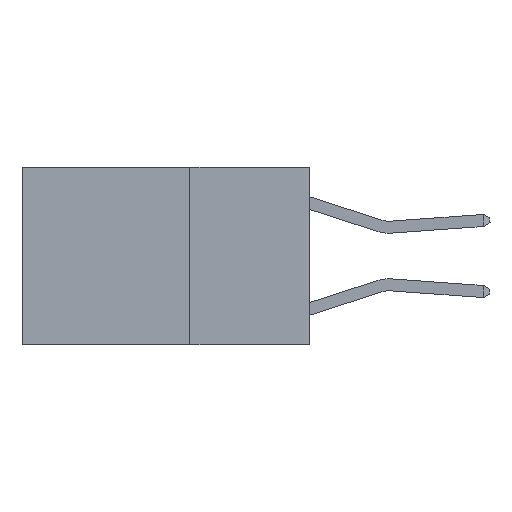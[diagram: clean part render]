
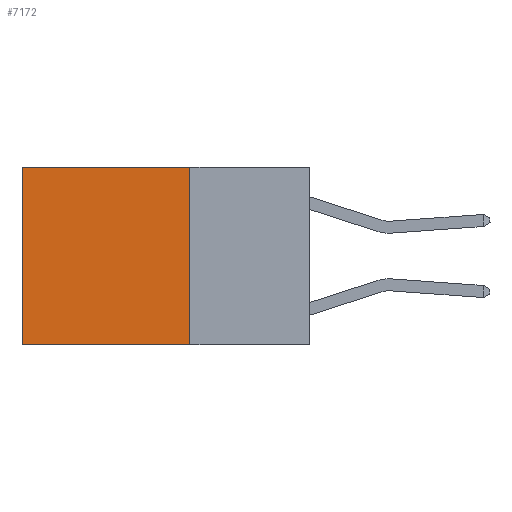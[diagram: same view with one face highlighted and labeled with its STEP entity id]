
A CAD part, left-side view. The second image highlights one B-rep face of the part: STEP entity #7172.
In plain terms, the highlighted planar face has unit normal (-1, 0, 0).
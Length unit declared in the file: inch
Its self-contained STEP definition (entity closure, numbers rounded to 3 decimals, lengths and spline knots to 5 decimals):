
#944 = ORIENTED_EDGE ( 'NONE', *, *, #3419, .T. ) ;
#1296 = LINE ( 'NONE', #1952, #4700 ) ;
#1952 = CARTESIAN_POINT ( 'NONE',  ( 0.2625, 0.25, 0. ) ) ;
#2015 = ORIENTED_EDGE ( 'NONE', *, *, #5008, .F. ) ;
#2053 = EDGE_CURVE ( 'NONE', #6786, #6449, #12035, .T. ) ;
#2470 = DIRECTION ( 'NONE',  ( 1., 0., 0. ) ) ;
#3419 = EDGE_CURVE ( 'NONE', #17197, #6449, #12396, .T. ) ;
#3831 = ORIENTED_EDGE ( 'NONE', *, *, #2053, .F. ) ;
#4368 = VERTEX_POINT ( 'NONE', #16659 ) ;
#4700 = VECTOR ( 'NONE', #11800, 39.37008 ) ;
#4838 = DIRECTION ( 'NONE',  ( 0., 0., -1. ) ) ;
#5008 = EDGE_CURVE ( 'NONE', #4368, #6786, #13356, .T. ) ;
#6449 = VERTEX_POINT ( 'NONE', #8469 ) ;
#6786 = VERTEX_POINT ( 'NONE', #12596 ) ;
#7172 = ADVANCED_FACE ( 'NONE', ( #14935 ), #10986, .F. ) ;
#8469 = CARTESIAN_POINT ( 'NONE',  ( 0.2625, 0.6, -0.37 ) ) ;
#9578 = EDGE_CURVE ( 'NONE', #4368, #17197, #1296, .T. ) ;
#9776 = AXIS2_PLACEMENT_3D ( 'NONE', #14959, #2470, #12339 ) ;
#10275 = ORIENTED_EDGE ( 'NONE', *, *, #9578, .T. ) ;
#10650 = CARTESIAN_POINT ( 'NONE',  ( 0.2625, 0.25, 0. ) ) ;
#10986 = PLANE ( 'NONE',  #9776 ) ;
#11800 = DIRECTION ( 'NONE',  ( 0., 1., 0. ) ) ;
#11935 = CARTESIAN_POINT ( 'NONE',  ( 0.2625, 0.25, -0.37 ) ) ;
#12035 = LINE ( 'NONE', #11935, #15172 ) ;
#12339 = DIRECTION ( 'NONE',  ( 0., 0., -1. ) ) ;
#12396 = LINE ( 'NONE', #14474, #16318 ) ;
#12596 = CARTESIAN_POINT ( 'NONE',  ( 0.2625, 0.25, -0.37 ) ) ;
#13356 = LINE ( 'NONE', #10650, #16847 ) ;
#14474 = CARTESIAN_POINT ( 'NONE',  ( 0.2625, 0.6, 0. ) ) ;
#14495 = EDGE_LOOP ( 'NONE', ( #944, #3831, #2015, #10275 ) ) ;
#14935 = FACE_OUTER_BOUND ( 'NONE', #14495, .T. ) ;
#14959 = CARTESIAN_POINT ( 'NONE',  ( 0.2625, 0.25, 0. ) ) ;
#15172 = VECTOR ( 'NONE', #15927, 39.37008 ) ;
#15873 = DIRECTION ( 'NONE',  ( 0., 0., -1. ) ) ;
#15927 = DIRECTION ( 'NONE',  ( 0., 1., 0. ) ) ;
#16318 = VECTOR ( 'NONE', #4838, 39.37008 ) ;
#16659 = CARTESIAN_POINT ( 'NONE',  ( 0.2625, 0.25, 0. ) ) ;
#16809 = CARTESIAN_POINT ( 'NONE',  ( 0.2625, 0.6, 0. ) ) ;
#16847 = VECTOR ( 'NONE', #15873, 39.37008 ) ;
#17197 = VERTEX_POINT ( 'NONE', #16809 ) ;
